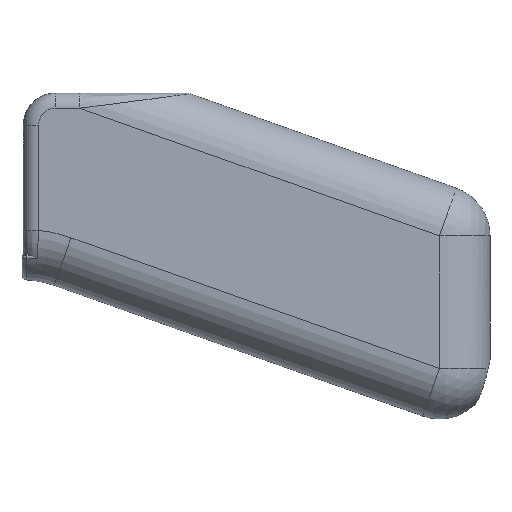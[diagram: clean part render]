
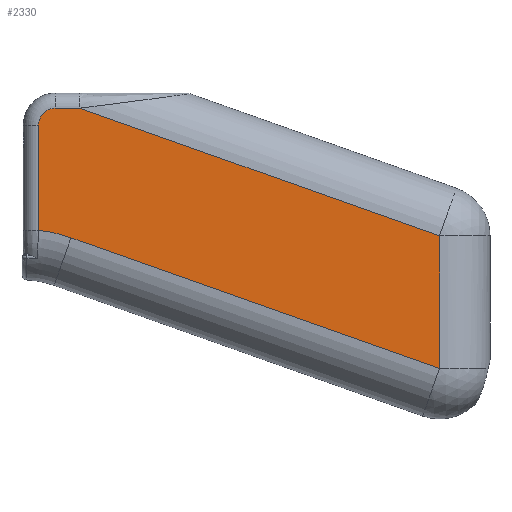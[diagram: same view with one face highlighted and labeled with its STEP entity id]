
A CAD part, left-side view. The second image highlights one B-rep face of the part: STEP entity #2330.
In plain terms, the highlighted planar face has unit normal (-1, 0, 0).
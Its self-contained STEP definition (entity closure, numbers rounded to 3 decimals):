
#26 = AXIS2_PLACEMENT_3D ( 'NONE', #1307, #2465, #740 ) ;
#42 = EDGE_CURVE ( 'NONE', #1191, #1562, #1161, .T. ) ;
#219 = VERTEX_POINT ( 'NONE', #2636 ) ;
#299 = VECTOR ( 'NONE', #2108, 1000. ) ;
#300 = ORIENTED_EDGE ( 'NONE', *, *, #620, .T. ) ;
#402 = CARTESIAN_POINT ( 'NONE',  ( 7.057, 0.864, -105.267 ) ) ;
#461 = DIRECTION ( 'NONE',  ( 0., 0., -1. ) ) ;
#462 = PLANE ( 'NONE',  #26 ) ;
#503 = CARTESIAN_POINT ( 'NONE',  ( 7.057, -5.74, -55.563 ) ) ;
#561 = CARTESIAN_POINT ( 'NONE',  ( 7.057, -81.855, -77.494 ) ) ;
#620 = EDGE_CURVE ( 'NONE', #219, #2380, #2166, .T. ) ;
#684 = DIRECTION ( 'NONE',  ( 0., 0., 1. ) ) ;
#689 = CARTESIAN_POINT ( 'NONE',  ( 7.057, 27.673, -52.213 ) ) ;
#731 = CARTESIAN_POINT ( 'NONE',  ( 7.057, -2.39, -55.563 ) ) ;
#740 = DIRECTION ( 'NONE',  ( 0., 0., 1. ) ) ;
#783 = DIRECTION ( 'NONE',  ( 0., 0., 1. ) ) ;
#888 = EDGE_LOOP ( 'NONE', ( #1892, #3092, #2196, #300, #1764, #2797, #2139 ) ) ;
#923 = VERTEX_POINT ( 'NONE', #731 ) ;
#1066 = LINE ( 'NONE', #689, #299 ) ;
#1137 = EDGE_CURVE ( 'NONE', #3076, #923, #2923, .T. ) ;
#1161 = LINE ( 'NONE', #1806, #2537 ) ;
#1191 = VERTEX_POINT ( 'NONE', #561 ) ;
#1266 = CARTESIAN_POINT ( 'NONE',  ( 7.057, -35.345, -87.282 ) ) ;
#1307 = CARTESIAN_POINT ( 'NONE',  ( 7.057, 27.673, 87.93 ) ) ;
#1339 = CIRCLE ( 'NONE', #3442, 29.05 ) ;
#1351 = VERTEX_POINT ( 'NONE', #3434 ) ;
#1486 = DIRECTION ( 'NONE',  ( 0., 0., 1. ) ) ;
#1562 = VERTEX_POINT ( 'NONE', #2534 ) ;
#1582 = CARTESIAN_POINT ( 'NONE',  ( 7.057, -2.39, 87.93 ) ) ;
#1609 = CARTESIAN_POINT ( 'NONE',  ( 7.057, -81.855, -103.769 ) ) ;
#1688 = EDGE_CURVE ( 'NONE', #1351, #219, #1339, .T. ) ;
#1764 = ORIENTED_EDGE ( 'NONE', *, *, #3699, .T. ) ;
#1793 = DIRECTION ( 'NONE',  ( 0., 0.943, 0.334 ) ) ;
#1806 = CARTESIAN_POINT ( 'NONE',  ( 7.057, -28.663, -58.638 ) ) ;
#1845 = CARTESIAN_POINT ( 'NONE',  ( 7.057, -81.855, 87.93 ) ) ;
#1850 = EDGE_CURVE ( 'NONE', #1562, #3076, #1066, .T. ) ;
#1892 = ORIENTED_EDGE ( 'NONE', *, *, #1137, .T. ) ;
#2062 = VECTOR ( 'NONE', #461, 1000. ) ;
#2108 = DIRECTION ( 'NONE',  ( 0., 1., 0. ) ) ;
#2139 = ORIENTED_EDGE ( 'NONE', *, *, #1850, .T. ) ;
#2166 = LINE ( 'NONE', #1266, #3628 ) ;
#2196 = ORIENTED_EDGE ( 'NONE', *, *, #1688, .T. ) ;
#2226 = AXIS2_PLACEMENT_3D ( 'NONE', #503, #2514, #783 ) ;
#2311 = CARTESIAN_POINT ( 'NONE',  ( 7.057, -5.74, -52.213 ) ) ;
#2330 = ADVANCED_FACE ( 'NONE', ( #2561 ), #462, .T. ) ;
#2380 = VERTEX_POINT ( 'NONE', #1609 ) ;
#2401 = DIRECTION ( 'NONE',  ( 1., 0., 0. ) ) ;
#2465 = DIRECTION ( 'NONE',  ( -1., 0., 0. ) ) ;
#2514 = DIRECTION ( 'NONE',  ( -1., 0., 0. ) ) ;
#2534 = CARTESIAN_POINT ( 'NONE',  ( 7.057, -10.538, -52.213 ) ) ;
#2537 = VECTOR ( 'NONE', #1793, 1000. ) ;
#2561 = FACE_OUTER_BOUND ( 'NONE', #888, .T. ) ;
#2636 = CARTESIAN_POINT ( 'NONE',  ( 7.057, -8.843, -77.887 ) ) ;
#2797 = ORIENTED_EDGE ( 'NONE', *, *, #42, .T. ) ;
#2923 = CIRCLE ( 'NONE', #2226, 3.35 ) ;
#3012 = DIRECTION ( 'NONE',  ( 0., -0.943, -0.334 ) ) ;
#3053 = VECTOR ( 'NONE', #1486, 1000. ) ;
#3076 = VERTEX_POINT ( 'NONE', #2311 ) ;
#3092 = ORIENTED_EDGE ( 'NONE', *, *, #3246, .T. ) ;
#3137 = LINE ( 'NONE', #1845, #3053 ) ;
#3246 = EDGE_CURVE ( 'NONE', #923, #1351, #3632, .T. ) ;
#3434 = CARTESIAN_POINT ( 'NONE',  ( 7.057, -2.39, -76.4 ) ) ;
#3442 = AXIS2_PLACEMENT_3D ( 'NONE', #402, #2401, #684 ) ;
#3628 = VECTOR ( 'NONE', #3012, 1000. ) ;
#3632 = LINE ( 'NONE', #1582, #2062 ) ;
#3699 = EDGE_CURVE ( 'NONE', #2380, #1191, #3137, .T. ) ;
